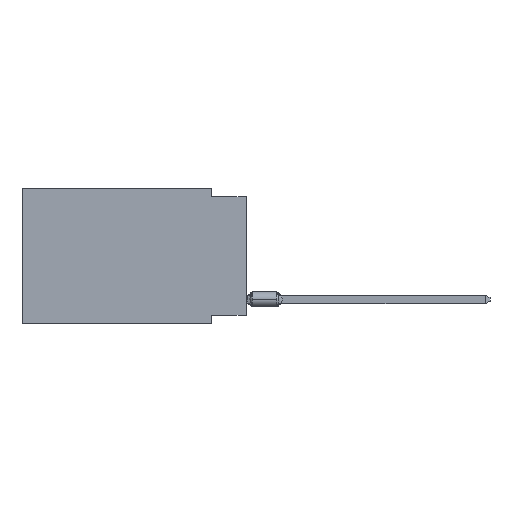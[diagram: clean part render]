
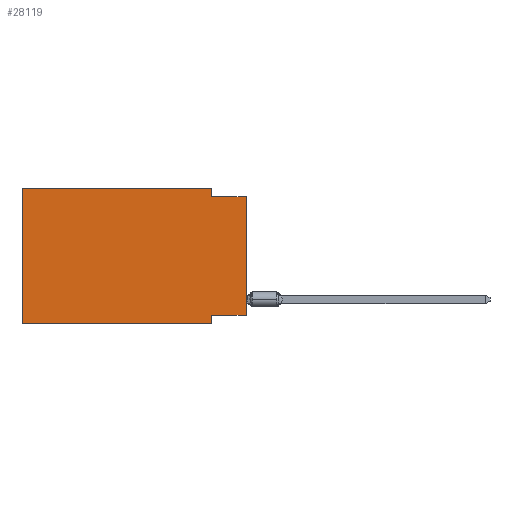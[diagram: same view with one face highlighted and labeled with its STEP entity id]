
A CAD part, left-side view. The second image highlights one B-rep face of the part: STEP entity #28119.
In plain terms, the highlighted planar face has unit normal (-1, 0, 0).
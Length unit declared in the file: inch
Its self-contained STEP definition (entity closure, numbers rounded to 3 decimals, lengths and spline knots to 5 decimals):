
#300 = LINE ( 'NONE', #20359, #20086 ) ;
#307 = CARTESIAN_POINT ( 'NONE',  ( 0., 0., -0.025 ) ) ;
#841 = VERTEX_POINT ( 'NONE', #8619 ) ;
#1064 = DIRECTION ( 'NONE',  ( 0., 0., 1. ) ) ;
#1373 = EDGE_CURVE ( 'NONE', #2024, #17857, #21496, .T. ) ;
#1523 = LINE ( 'NONE', #8644, #9197 ) ;
#1858 = CARTESIAN_POINT ( 'NONE',  ( 0., 0.645, -0.39 ) ) ;
#2024 = VERTEX_POINT ( 'NONE', #26233 ) ;
#2106 = VECTOR ( 'NONE', #1064, 39.37008 ) ;
#2867 = ORIENTED_EDGE ( 'NONE', *, *, #23115, .F. ) ;
#3858 = VECTOR ( 'NONE', #6083, 39.37008 ) ;
#3897 = CARTESIAN_POINT ( 'NONE',  ( 0., 0., -0.365 ) ) ;
#4366 = CARTESIAN_POINT ( 'NONE',  ( 0., 0.1, -0.39 ) ) ;
#4382 = EDGE_CURVE ( 'NONE', #19836, #841, #23212, .T. ) ;
#4961 = CARTESIAN_POINT ( 'NONE',  ( 0., 0.645, 0. ) ) ;
#5900 = ORIENTED_EDGE ( 'NONE', *, *, #19548, .F. ) ;
#6083 = DIRECTION ( 'NONE',  ( 0., -1., 0. ) ) ;
#6136 = VECTOR ( 'NONE', #24992, 39.37008 ) ;
#6448 = VECTOR ( 'NONE', #16662, 39.37008 ) ;
#6784 = CARTESIAN_POINT ( 'NONE',  ( 0., 0.1, -0.39 ) ) ;
#7117 = LINE ( 'NONE', #12613, #8738 ) ;
#7694 = CARTESIAN_POINT ( 'NONE',  ( 0., 0.1, -0.025 ) ) ;
#7875 = LINE ( 'NONE', #30511, #3858 ) ;
#7988 = VERTEX_POINT ( 'NONE', #307 ) ;
#8065 = DIRECTION ( 'NONE',  ( 0., 0., 1. ) ) ;
#8619 = CARTESIAN_POINT ( 'NONE',  ( 0., 0.645, 0. ) ) ;
#8644 = CARTESIAN_POINT ( 'NONE',  ( 0., 0., -0.025 ) ) ;
#8738 = VECTOR ( 'NONE', #22939, 39.37008 ) ;
#9197 = VECTOR ( 'NONE', #31114, 39.37008 ) ;
#11261 = CARTESIAN_POINT ( 'NONE',  ( 0., 0.645, 0. ) ) ;
#11845 = AXIS2_PLACEMENT_3D ( 'NONE', #24846, #17577, #12100 ) ;
#12100 = DIRECTION ( 'NONE',  ( 0., 0., -1. ) ) ;
#12467 = EDGE_CURVE ( 'NONE', #19836, #17857, #7875, .T. ) ;
#12613 = CARTESIAN_POINT ( 'NONE',  ( 0., 0., -0.365 ) ) ;
#13509 = ORIENTED_EDGE ( 'NONE', *, *, #29371, .F. ) ;
#15849 = VERTEX_POINT ( 'NONE', #7694 ) ;
#16033 = DIRECTION ( 'NONE',  ( 0., 0., -1. ) ) ;
#16662 = DIRECTION ( 'NONE',  ( 0., 0., -1. ) ) ;
#17085 = EDGE_CURVE ( 'NONE', #15849, #7988, #1523, .T. ) ;
#17246 = CARTESIAN_POINT ( 'NONE',  ( 0., 0.1, 0. ) ) ;
#17577 = DIRECTION ( 'NONE',  ( 1., 0., 0. ) ) ;
#17857 = VERTEX_POINT ( 'NONE', #4366 ) ;
#17949 = ORIENTED_EDGE ( 'NONE', *, *, #1373, .F. ) ;
#18217 = EDGE_LOOP ( 'NONE', ( #29420, #24013, #2867, #5900, #31945, #19675, #17949, #13509 ) ) ;
#19371 = PLANE ( 'NONE',  #11845 ) ;
#19548 = EDGE_CURVE ( 'NONE', #841, #20928, #26471, .T. ) ;
#19675 = ORIENTED_EDGE ( 'NONE', *, *, #12467, .T. ) ;
#19836 = VERTEX_POINT ( 'NONE', #1858 ) ;
#20086 = VECTOR ( 'NONE', #8065, 39.37008 ) ;
#20359 = CARTESIAN_POINT ( 'NONE',  ( 0., 0., 0. ) ) ;
#20928 = VERTEX_POINT ( 'NONE', #17246 ) ;
#21496 = LINE ( 'NONE', #6784, #6448 ) ;
#22939 = DIRECTION ( 'NONE',  ( 0., 1., 0. ) ) ;
#23115 = EDGE_CURVE ( 'NONE', #20928, #15849, #23443, .T. ) ;
#23212 = LINE ( 'NONE', #11261, #2106 ) ;
#23443 = LINE ( 'NONE', #26028, #29694 ) ;
#24013 = ORIENTED_EDGE ( 'NONE', *, *, #17085, .F. ) ;
#24846 = CARTESIAN_POINT ( 'NONE',  ( 0., 0.645, 0. ) ) ;
#24992 = DIRECTION ( 'NONE',  ( 0., -1., 0. ) ) ;
#25411 = VERTEX_POINT ( 'NONE', #3897 ) ;
#26028 = CARTESIAN_POINT ( 'NONE',  ( 0., 0.1, 0. ) ) ;
#26233 = CARTESIAN_POINT ( 'NONE',  ( 0., 0.1, -0.365 ) ) ;
#26471 = LINE ( 'NONE', #4961, #6136 ) ;
#27272 = FACE_OUTER_BOUND ( 'NONE', #18217, .T. ) ;
#28119 = ADVANCED_FACE ( 'NONE', ( #27272 ), #19371, .F. ) ;
#29371 = EDGE_CURVE ( 'NONE', #25411, #2024, #7117, .T. ) ;
#29404 = EDGE_CURVE ( 'NONE', #25411, #7988, #300, .T. ) ;
#29420 = ORIENTED_EDGE ( 'NONE', *, *, #29404, .T. ) ;
#29694 = VECTOR ( 'NONE', #16033, 39.37008 ) ;
#30511 = CARTESIAN_POINT ( 'NONE',  ( 0., 0.645, -0.39 ) ) ;
#31114 = DIRECTION ( 'NONE',  ( 0., -1., 0. ) ) ;
#31945 = ORIENTED_EDGE ( 'NONE', *, *, #4382, .F. ) ;
